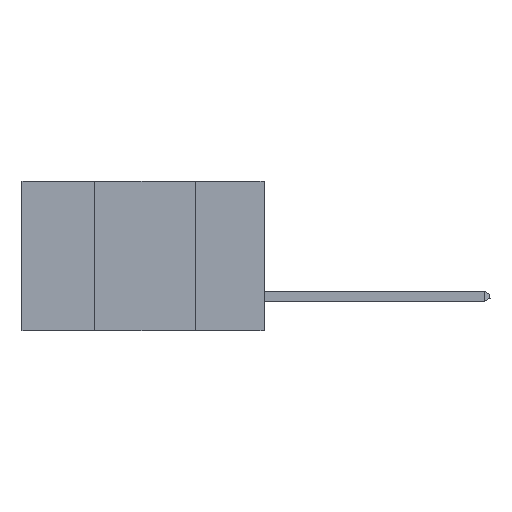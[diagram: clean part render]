
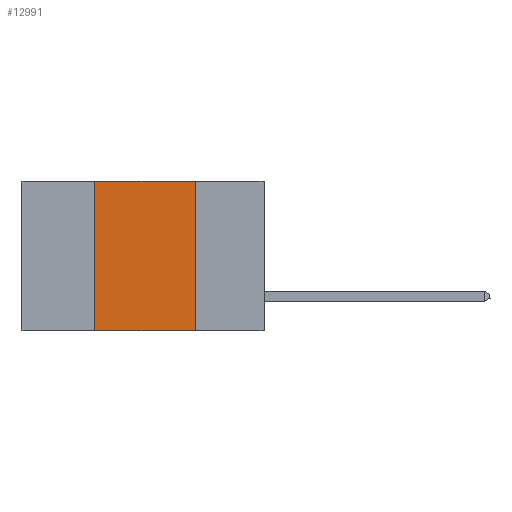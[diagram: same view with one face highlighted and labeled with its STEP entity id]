
A CAD part, left-side view. The second image highlights one B-rep face of the part: STEP entity #12991.
In plain terms, the highlighted planar face has unit normal (-1, 0, 0).
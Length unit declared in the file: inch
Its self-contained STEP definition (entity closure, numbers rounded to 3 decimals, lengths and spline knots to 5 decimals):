
#122 = DIRECTION ( 'NONE',  ( 0., 0., -1. ) ) ;
#446 = ORIENTED_EDGE ( 'NONE', *, *, #11592, .T. ) ;
#694 = CARTESIAN_POINT ( 'NONE',  ( 0., 0.42, 0. ) ) ;
#2705 = EDGE_CURVE ( 'NONE', #21417, #2849, #21368, .T. ) ;
#2849 = VERTEX_POINT ( 'NONE', #7422 ) ;
#2985 = CARTESIAN_POINT ( 'NONE',  ( 0., 0.42, -0.37 ) ) ;
#3457 = EDGE_CURVE ( 'NONE', #15451, #8428, #9182, .T. ) ;
#6255 = CARTESIAN_POINT ( 'NONE',  ( 0., 0.6, 0. ) ) ;
#7422 = CARTESIAN_POINT ( 'NONE',  ( 0., 0.17, -0.37 ) ) ;
#8060 = EDGE_LOOP ( 'NONE', ( #13274, #11270, #20624, #446 ) ) ;
#8334 = DIRECTION ( 'NONE',  ( 1., 0., 0. ) ) ;
#8428 = VERTEX_POINT ( 'NONE', #22393 ) ;
#8802 = CARTESIAN_POINT ( 'NONE',  ( 0., 0.17, 0. ) ) ;
#8922 = VECTOR ( 'NONE', #10907, 39.37008 ) ;
#9182 = LINE ( 'NONE', #694, #12132 ) ;
#10796 = CARTESIAN_POINT ( 'NONE',  ( 0., 0.6, -0.37 ) ) ;
#10907 = DIRECTION ( 'NONE',  ( 0., 0., -1. ) ) ;
#10947 = DIRECTION ( 'NONE',  ( 0., 0., 1. ) ) ;
#11270 = ORIENTED_EDGE ( 'NONE', *, *, #13763, .F. ) ;
#11416 = CARTESIAN_POINT ( 'NONE',  ( 0., 0.17, 0. ) ) ;
#11592 = EDGE_CURVE ( 'NONE', #15451, #2849, #17639, .T. ) ;
#12132 = VECTOR ( 'NONE', #10947, 39.37008 ) ;
#12991 = ADVANCED_FACE ( 'NONE', ( #20505 ), #20893, .F. ) ;
#13274 = ORIENTED_EDGE ( 'NONE', *, *, #2705, .F. ) ;
#13658 = AXIS2_PLACEMENT_3D ( 'NONE', #6255, #8334, #122 ) ;
#13763 = EDGE_CURVE ( 'NONE', #8428, #21417, #25999, .T. ) ;
#15451 = VERTEX_POINT ( 'NONE', #2985 ) ;
#16502 = CARTESIAN_POINT ( 'NONE',  ( 0., 0.6, 0. ) ) ;
#16599 = DIRECTION ( 'NONE',  ( 0., -1., 0. ) ) ;
#17639 = LINE ( 'NONE', #10796, #23489 ) ;
#18947 = DIRECTION ( 'NONE',  ( 0., -1., 0. ) ) ;
#19494 = VECTOR ( 'NONE', #16599, 39.37008 ) ;
#20505 = FACE_OUTER_BOUND ( 'NONE', #8060, .T. ) ;
#20624 = ORIENTED_EDGE ( 'NONE', *, *, #3457, .F. ) ;
#20893 = PLANE ( 'NONE',  #13658 ) ;
#21368 = LINE ( 'NONE', #8802, #8922 ) ;
#21417 = VERTEX_POINT ( 'NONE', #11416 ) ;
#22393 = CARTESIAN_POINT ( 'NONE',  ( 0., 0.42, 0. ) ) ;
#23489 = VECTOR ( 'NONE', #18947, 39.37008 ) ;
#25999 = LINE ( 'NONE', #16502, #19494 ) ;
